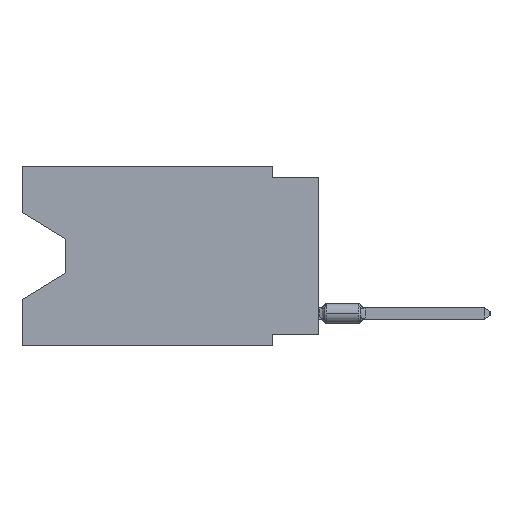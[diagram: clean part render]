
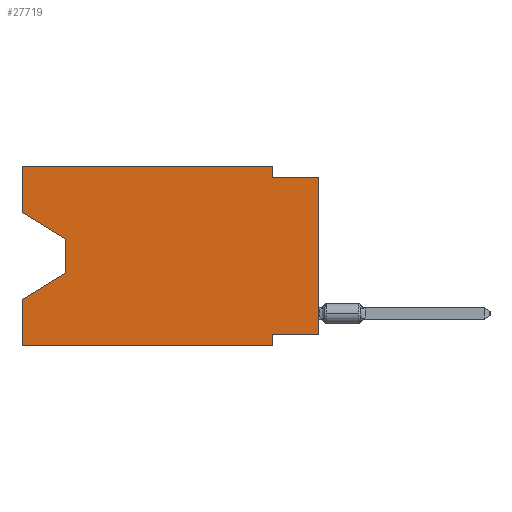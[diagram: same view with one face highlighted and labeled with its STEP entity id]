
A CAD part, left-side view. The second image highlights one B-rep face of the part: STEP entity #27719.
In plain terms, the highlighted planar face has unit normal (-1, 0, 0).
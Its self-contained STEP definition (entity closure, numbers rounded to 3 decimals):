
#658 = DIRECTION ( 'NONE',  ( 0., 0., -1. ) ) ;
#1077 = VECTOR ( 'NONE', #30942, 1000. ) ;
#1435 = VERTEX_POINT ( 'NONE', #15257 ) ;
#1535 = EDGE_CURVE ( 'NONE', #22477, #4515, #15063, .T. ) ;
#2280 = ORIENTED_EDGE ( 'NONE', *, *, #33403, .T. ) ;
#2653 = ORIENTED_EDGE ( 'NONE', *, *, #14939, .T. ) ;
#3356 = VECTOR ( 'NONE', #25006, 1000. ) ;
#3980 = CARTESIAN_POINT ( 'NONE',  ( 0., 16.383, 0. ) ) ;
#4034 = DIRECTION ( 'NONE',  ( 0., -0.855, -0.519 ) ) ;
#4229 = CARTESIAN_POINT ( 'NONE',  ( 0., 16.383, -9.906 ) ) ;
#4515 = VERTEX_POINT ( 'NONE', #6039 ) ;
#5054 = ORIENTED_EDGE ( 'NONE', *, *, #36134, .F. ) ;
#5495 = EDGE_CURVE ( 'NONE', #34434, #25968, #9122, .T. ) ;
#6039 = CARTESIAN_POINT ( 'NONE',  ( 0., 2.54, -0.635 ) ) ;
#6284 = CARTESIAN_POINT ( 'NONE',  ( 0., 16.383, 0. ) ) ;
#7940 = VECTOR ( 'NONE', #9296, 1000. ) ;
#7974 = CARTESIAN_POINT ( 'NONE',  ( 0., 16.383, 0. ) ) ;
#8489 = DIRECTION ( 'NONE',  ( 0., -1., 0. ) ) ;
#8782 = VECTOR ( 'NONE', #8489, 1000. ) ;
#9122 = LINE ( 'NONE', #6284, #13206 ) ;
#9296 = DIRECTION ( 'NONE',  ( 0., 0., 1. ) ) ;
#9516 = CARTESIAN_POINT ( 'NONE',  ( 0., 2.54, -9.906 ) ) ;
#9681 = LINE ( 'NONE', #23922, #7940 ) ;
#9734 = VECTOR ( 'NONE', #9743, 1000. ) ;
#9743 = DIRECTION ( 'NONE',  ( 0., 1., 0. ) ) ;
#9923 = CARTESIAN_POINT ( 'NONE',  ( 0., 0., -9.271 ) ) ;
#10128 = CARTESIAN_POINT ( 'NONE',  ( 0., 16.383, -2.546 ) ) ;
#10723 = AXIS2_PLACEMENT_3D ( 'NONE', #3980, #23905, #27131 ) ;
#10882 = ORIENTED_EDGE ( 'NONE', *, *, #12410, .F. ) ;
#11261 = EDGE_LOOP ( 'NONE', ( #2653, #12202, #22897, #29630, #2280, #32850, #10882, #20246, #28040, #30736, #16646, #5054 ) ) ;
#11267 = CARTESIAN_POINT ( 'NONE',  ( 0., 0., -9.271 ) ) ;
#11825 = VERTEX_POINT ( 'NONE', #33613 ) ;
#11990 = EDGE_CURVE ( 'NONE', #24177, #25968, #20167, .T. ) ;
#12202 = ORIENTED_EDGE ( 'NONE', *, *, #37227, .T. ) ;
#12410 = EDGE_CURVE ( 'NONE', #36570, #1435, #32705, .T. ) ;
#12723 = VECTOR ( 'NONE', #14850, 1000. ) ;
#13206 = VECTOR ( 'NONE', #18247, 1000. ) ;
#14006 = LINE ( 'NONE', #31815, #30183 ) ;
#14018 = LINE ( 'NONE', #35040, #8782 ) ;
#14828 = CARTESIAN_POINT ( 'NONE',  ( 0., 13.97, -5.893 ) ) ;
#14850 = DIRECTION ( 'NONE',  ( 0., 0.855, -0.519 ) ) ;
#14939 = EDGE_CURVE ( 'NONE', #23241, #35918, #18448, .T. ) ;
#15063 = LINE ( 'NONE', #26637, #20060 ) ;
#15257 = CARTESIAN_POINT ( 'NONE',  ( 0., 2.54, -9.271 ) ) ;
#16584 = CARTESIAN_POINT ( 'NONE',  ( 0., 16.383, 0. ) ) ;
#16646 = ORIENTED_EDGE ( 'NONE', *, *, #27428, .F. ) ;
#17391 = VERTEX_POINT ( 'NONE', #16584 ) ;
#17515 = LINE ( 'NONE', #9516, #31272 ) ;
#18247 = DIRECTION ( 'NONE',  ( 0., 0., 1. ) ) ;
#18360 = VECTOR ( 'NONE', #35417, 1000. ) ;
#18448 = LINE ( 'NONE', #30019, #35912 ) ;
#20060 = VECTOR ( 'NONE', #658, 1000. ) ;
#20167 = LINE ( 'NONE', #23365, #12723 ) ;
#20246 = ORIENTED_EDGE ( 'NONE', *, *, #21607, .T. ) ;
#21064 = PLANE ( 'NONE',  #10723 ) ;
#21401 = CARTESIAN_POINT ( 'NONE',  ( 0., 0., -0.635 ) ) ;
#21573 = LINE ( 'NONE', #21401, #18360 ) ;
#21607 = EDGE_CURVE ( 'NONE', #36570, #11825, #9681, .T. ) ;
#21794 = LINE ( 'NONE', #27856, #3356 ) ;
#22477 = VERTEX_POINT ( 'NONE', #35337 ) ;
#22868 = CARTESIAN_POINT ( 'NONE',  ( 0., 2.54, -9.906 ) ) ;
#22897 = ORIENTED_EDGE ( 'NONE', *, *, #11990, .T. ) ;
#23241 = VERTEX_POINT ( 'NONE', #10128 ) ;
#23365 = CARTESIAN_POINT ( 'NONE',  ( 0., 13.97, -5.893 ) ) ;
#23514 = EDGE_CURVE ( 'NONE', #4515, #11825, #21573, .T. ) ;
#23905 = DIRECTION ( 'NONE',  ( 1., 0., 0. ) ) ;
#23922 = CARTESIAN_POINT ( 'NONE',  ( 0., 0., 0. ) ) ;
#24177 = VERTEX_POINT ( 'NONE', #14828 ) ;
#25006 = DIRECTION ( 'NONE',  ( 0., 0., -1. ) ) ;
#25748 = DIRECTION ( 'NONE',  ( 0., 0., 1. ) ) ;
#25968 = VERTEX_POINT ( 'NONE', #27863 ) ;
#26054 = DIRECTION ( 'NONE',  ( 0., 0., -1. ) ) ;
#26637 = CARTESIAN_POINT ( 'NONE',  ( 0., 2.54, 0. ) ) ;
#27131 = DIRECTION ( 'NONE',  ( 0., 0., -1. ) ) ;
#27428 = EDGE_CURVE ( 'NONE', #17391, #22477, #29558, .T. ) ;
#27719 = ADVANCED_FACE ( 'NONE', ( #35276 ), #21064, .F. ) ;
#27856 = CARTESIAN_POINT ( 'NONE',  ( 0., 13.97, -4.013 ) ) ;
#27864 = EDGE_CURVE ( 'NONE', #1435, #31998, #17515, .T. ) ;
#27863 = CARTESIAN_POINT ( 'NONE',  ( 0., 16.383, -7.36 ) ) ;
#28040 = ORIENTED_EDGE ( 'NONE', *, *, #23514, .F. ) ;
#29218 = CARTESIAN_POINT ( 'NONE',  ( 0., 13.97, -4.013 ) ) ;
#29558 = LINE ( 'NONE', #7974, #1077 ) ;
#29630 = ORIENTED_EDGE ( 'NONE', *, *, #5495, .F. ) ;
#30019 = CARTESIAN_POINT ( 'NONE',  ( 0., 16.383, -2.546 ) ) ;
#30183 = VECTOR ( 'NONE', #25748, 1000. ) ;
#30736 = ORIENTED_EDGE ( 'NONE', *, *, #1535, .F. ) ;
#30942 = DIRECTION ( 'NONE',  ( 0., -1., 0. ) ) ;
#31272 = VECTOR ( 'NONE', #26054, 1000. ) ;
#31815 = CARTESIAN_POINT ( 'NONE',  ( 0., 16.383, 0. ) ) ;
#31998 = VERTEX_POINT ( 'NONE', #22868 ) ;
#32705 = LINE ( 'NONE', #9923, #9734 ) ;
#32850 = ORIENTED_EDGE ( 'NONE', *, *, #27864, .F. ) ;
#33403 = EDGE_CURVE ( 'NONE', #34434, #31998, #14018, .T. ) ;
#33613 = CARTESIAN_POINT ( 'NONE',  ( 0., 0., -0.635 ) ) ;
#34434 = VERTEX_POINT ( 'NONE', #4229 ) ;
#35040 = CARTESIAN_POINT ( 'NONE',  ( 0., 16.383, -9.906 ) ) ;
#35276 = FACE_OUTER_BOUND ( 'NONE', #11261, .T. ) ;
#35337 = CARTESIAN_POINT ( 'NONE',  ( 0., 2.54, 0. ) ) ;
#35417 = DIRECTION ( 'NONE',  ( 0., -1., 0. ) ) ;
#35912 = VECTOR ( 'NONE', #4034, 1000. ) ;
#35918 = VERTEX_POINT ( 'NONE', #29218 ) ;
#36134 = EDGE_CURVE ( 'NONE', #23241, #17391, #14006, .T. ) ;
#36570 = VERTEX_POINT ( 'NONE', #11267 ) ;
#37227 = EDGE_CURVE ( 'NONE', #35918, #24177, #21794, .T. ) ;
